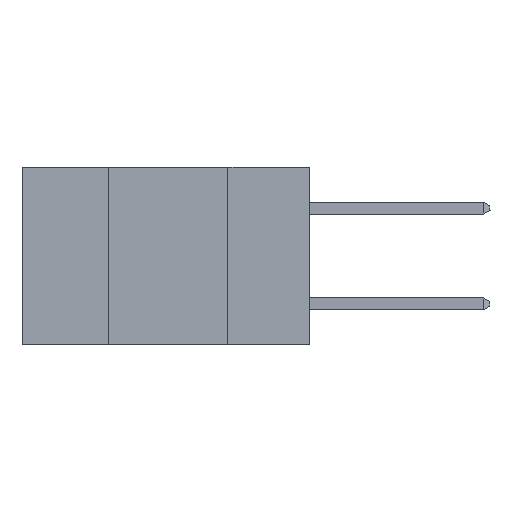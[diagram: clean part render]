
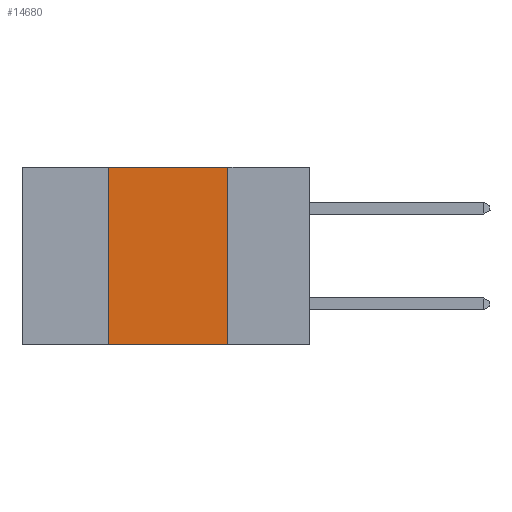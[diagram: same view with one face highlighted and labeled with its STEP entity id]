
A CAD part, left-side view. The second image highlights one B-rep face of the part: STEP entity #14680.
In plain terms, the highlighted planar face has unit normal (-1, 0, 0).
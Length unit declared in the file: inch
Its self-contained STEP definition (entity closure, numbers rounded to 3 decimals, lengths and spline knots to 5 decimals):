
#382 = VERTEX_POINT ( 'NONE', #2249 ) ;
#566 = CARTESIAN_POINT ( 'NONE',  ( 0., 0.42, -0.37 ) ) ;
#2249 = CARTESIAN_POINT ( 'NONE',  ( 0., 0.17, 0. ) ) ;
#3424 = ORIENTED_EDGE ( 'NONE', *, *, #24905, .F. ) ;
#4058 = EDGE_LOOP ( 'NONE', ( #3424, #21948, #11896, #5539 ) ) ;
#4139 = DIRECTION ( 'NONE',  ( 1., 0., 0. ) ) ;
#4454 = LINE ( 'NONE', #18390, #13988 ) ;
#4466 = EDGE_CURVE ( 'NONE', #18288, #15395, #15150, .T. ) ;
#5539 = ORIENTED_EDGE ( 'NONE', *, *, #4466, .T. ) ;
#7408 = CARTESIAN_POINT ( 'NONE',  ( 0., 0.42, 0. ) ) ;
#7933 = CARTESIAN_POINT ( 'NONE',  ( 0., 0.6, 0. ) ) ;
#8915 = CARTESIAN_POINT ( 'NONE',  ( 0., 0.6, -0.37 ) ) ;
#9567 = VECTOR ( 'NONE', #21601, 39.37008 ) ;
#11896 = ORIENTED_EDGE ( 'NONE', *, *, #20585, .F. ) ;
#11958 = CARTESIAN_POINT ( 'NONE',  ( 0., 0.42, 0. ) ) ;
#12248 = DIRECTION ( 'NONE',  ( 0., -1., 0. ) ) ;
#13988 = VECTOR ( 'NONE', #12248, 39.37008 ) ;
#14062 = VECTOR ( 'NONE', #20764, 39.37008 ) ;
#14680 = ADVANCED_FACE ( 'NONE', ( #17813 ), #16360, .F. ) ;
#15150 = LINE ( 'NONE', #8915, #14062 ) ;
#15337 = LINE ( 'NONE', #19655, #9567 ) ;
#15395 = VERTEX_POINT ( 'NONE', #15536 ) ;
#15536 = CARTESIAN_POINT ( 'NONE',  ( 0., 0.17, -0.37 ) ) ;
#16360 = PLANE ( 'NONE',  #18027 ) ;
#17813 = FACE_OUTER_BOUND ( 'NONE', #4058, .T. ) ;
#18027 = AXIS2_PLACEMENT_3D ( 'NONE', #7933, #4139, #20292 ) ;
#18288 = VERTEX_POINT ( 'NONE', #566 ) ;
#18390 = CARTESIAN_POINT ( 'NONE',  ( 0., 0.6, 0. ) ) ;
#18847 = EDGE_CURVE ( 'NONE', #19632, #382, #4454, .T. ) ;
#19632 = VERTEX_POINT ( 'NONE', #7408 ) ;
#19655 = CARTESIAN_POINT ( 'NONE',  ( 0., 0.17, 0. ) ) ;
#20292 = DIRECTION ( 'NONE',  ( 0., 0., -1. ) ) ;
#20585 = EDGE_CURVE ( 'NONE', #18288, #19632, #22278, .T. ) ;
#20764 = DIRECTION ( 'NONE',  ( 0., -1., 0. ) ) ;
#21601 = DIRECTION ( 'NONE',  ( 0., 0., -1. ) ) ;
#21948 = ORIENTED_EDGE ( 'NONE', *, *, #18847, .F. ) ;
#21988 = VECTOR ( 'NONE', #24235, 39.37008 ) ;
#22278 = LINE ( 'NONE', #11958, #21988 ) ;
#24235 = DIRECTION ( 'NONE',  ( 0., 0., 1. ) ) ;
#24905 = EDGE_CURVE ( 'NONE', #382, #15395, #15337, .T. ) ;
